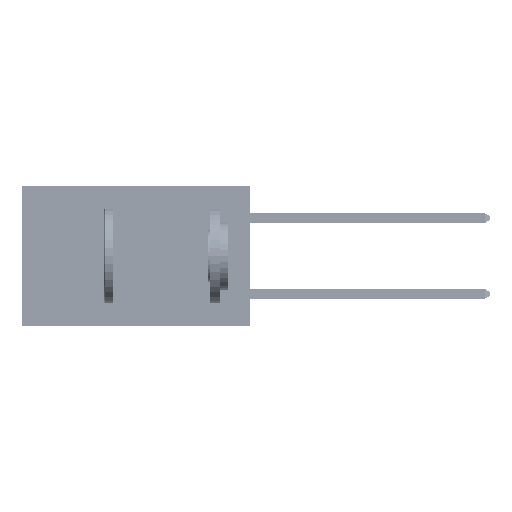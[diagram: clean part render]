
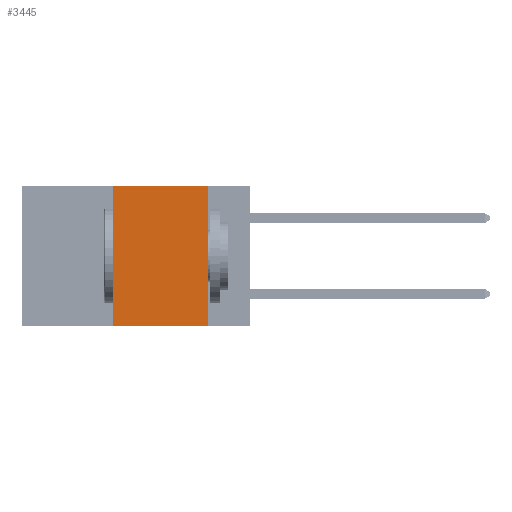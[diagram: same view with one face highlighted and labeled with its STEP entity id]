
A CAD part, left-side view. The second image highlights one B-rep face of the part: STEP entity #3445.
In plain terms, the highlighted planar face has unit normal (-1, 0, 0).
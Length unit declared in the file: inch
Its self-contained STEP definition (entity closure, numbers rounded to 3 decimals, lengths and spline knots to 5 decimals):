
#221 = DIRECTION ( 'NONE',  ( 0., 0., 1. ) ) ;
#3445 = ADVANCED_FACE ( 'NONE', ( #5202 ), #39699, .F. ) ;
#5202 = FACE_OUTER_BOUND ( 'NONE', #36285, .T. ) ;
#6354 = EDGE_CURVE ( 'NONE', #44012, #7069, #49540, .T. ) ;
#7069 = VERTEX_POINT ( 'NONE', #24969 ) ;
#7130 = ORIENTED_EDGE ( 'NONE', *, *, #6354, .F. ) ;
#8204 = CARTESIAN_POINT ( 'NONE',  ( 0., 0.6, 0. ) ) ;
#13192 = VECTOR ( 'NONE', #45279, 39.37008 ) ;
#16005 = VECTOR ( 'NONE', #25952, 39.37008 ) ;
#16019 = DIRECTION ( 'NONE',  ( 0., 0., -1. ) ) ;
#16165 = CARTESIAN_POINT ( 'NONE',  ( 0., 0.36, -0.37 ) ) ;
#17965 = VERTEX_POINT ( 'NONE', #47043 ) ;
#18008 = CARTESIAN_POINT ( 'NONE',  ( 0., 0.6, 0. ) ) ;
#22045 = ORIENTED_EDGE ( 'NONE', *, *, #42767, .F. ) ;
#24177 = VECTOR ( 'NONE', #221, 39.37008 ) ;
#24969 = CARTESIAN_POINT ( 'NONE',  ( 0., 0.36, 0. ) ) ;
#25952 = DIRECTION ( 'NONE',  ( 0., -1., 0. ) ) ;
#26059 = CARTESIAN_POINT ( 'NONE',  ( 0., 0.11, -0.37 ) ) ;
#26808 = ORIENTED_EDGE ( 'NONE', *, *, #46192, .T. ) ;
#27009 = VECTOR ( 'NONE', #42958, 39.37008 ) ;
#33982 = CARTESIAN_POINT ( 'NONE',  ( 0., 0.6, -0.37 ) ) ;
#34284 = AXIS2_PLACEMENT_3D ( 'NONE', #8204, #35542, #16019 ) ;
#35542 = DIRECTION ( 'NONE',  ( 1., 0., 0. ) ) ;
#35782 = LINE ( 'NONE', #18008, #16005 ) ;
#36285 = EDGE_LOOP ( 'NONE', ( #42395, #22045, #7130, #26808 ) ) ;
#39699 = PLANE ( 'NONE',  #34284 ) ;
#40447 = LINE ( 'NONE', #33982, #13192 ) ;
#42395 = ORIENTED_EDGE ( 'NONE', *, *, #44293, .F. ) ;
#42767 = EDGE_CURVE ( 'NONE', #7069, #17965, #35782, .T. ) ;
#42958 = DIRECTION ( 'NONE',  ( 0., 0., -1. ) ) ;
#44012 = VERTEX_POINT ( 'NONE', #16165 ) ;
#44293 = EDGE_CURVE ( 'NONE', #17965, #45584, #51195, .T. ) ;
#45279 = DIRECTION ( 'NONE',  ( 0., -1., 0. ) ) ;
#45584 = VERTEX_POINT ( 'NONE', #26059 ) ;
#46192 = EDGE_CURVE ( 'NONE', #44012, #45584, #40447, .T. ) ;
#47043 = CARTESIAN_POINT ( 'NONE',  ( 0., 0.11, 0. ) ) ;
#47674 = CARTESIAN_POINT ( 'NONE',  ( 0., 0.36, 0. ) ) ;
#49540 = LINE ( 'NONE', #47674, #24177 ) ;
#50783 = CARTESIAN_POINT ( 'NONE',  ( 0., 0.11, 0. ) ) ;
#51195 = LINE ( 'NONE', #50783, #27009 ) ;
